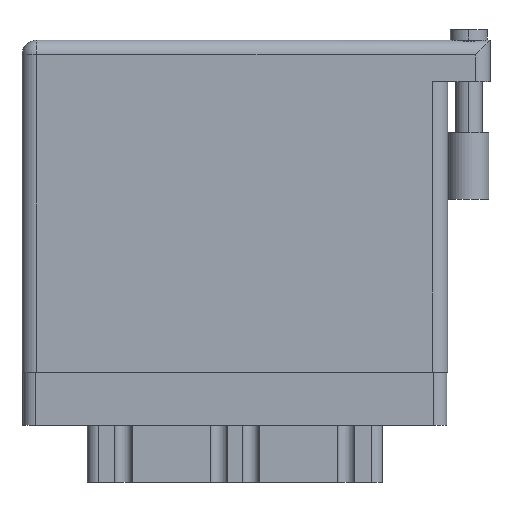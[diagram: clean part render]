
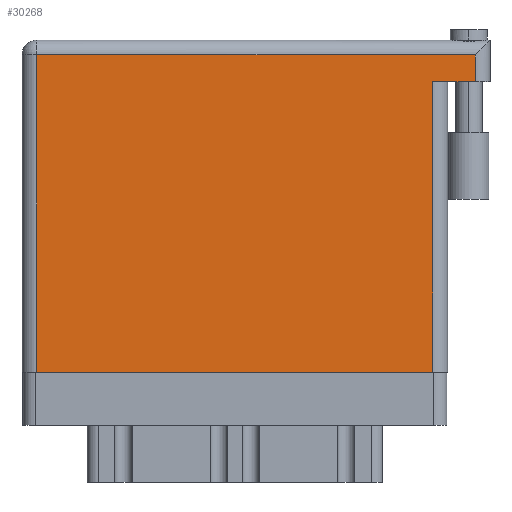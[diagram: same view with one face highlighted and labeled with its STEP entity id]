
A CAD part, front view. The second image highlights one B-rep face of the part: STEP entity #30268.
In plain terms, the highlighted face is planar.
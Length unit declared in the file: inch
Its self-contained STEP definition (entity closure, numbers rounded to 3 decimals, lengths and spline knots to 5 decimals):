
#124 = ORIENTED_EDGE ( 'NONE', *, *, #16181, .T. ) ;
#976 = DIRECTION ( 'NONE',  ( 0., 1., 0. ) ) ;
#1570 = VECTOR ( 'NONE', #4460, 39.37008 ) ;
#2046 = VECTOR ( 'NONE', #31741, 39.37008 ) ;
#2298 = LINE ( 'NONE', #10660, #4826 ) ;
#2504 = ORIENTED_EDGE ( 'NONE', *, *, #26879, .T. ) ;
#2647 = VERTEX_POINT ( 'NONE', #14250 ) ;
#3140 = ORIENTED_EDGE ( 'NONE', *, *, #25198, .T. ) ;
#3285 = VERTEX_POINT ( 'NONE', #3614 ) ;
#3614 = CARTESIAN_POINT ( 'NONE',  ( 2.138, 1.496, 0. ) ) ;
#4226 = EDGE_CURVE ( 'NONE', #24321, #3285, #29999, .T. ) ;
#4243 = CARTESIAN_POINT ( 'NONE',  ( 0., 1.566, 0. ) ) ;
#4258 = VERTEX_POINT ( 'NONE', #6030 ) ;
#4420 = DIRECTION ( 'NONE',  ( -1., 0., 0. ) ) ;
#4460 = DIRECTION ( 'NONE',  ( 1., 0., 0. ) ) ;
#4727 = CARTESIAN_POINT ( 'NONE',  ( 1.938, 1.369, 0. ) ) ;
#4826 = VECTOR ( 'NONE', #28879, 39.37008 ) ;
#6030 = CARTESIAN_POINT ( 'NONE',  ( 0.07, 0., 0. ) ) ;
#8004 = VECTOR ( 'NONE', #25530, 39.37008 ) ;
#8796 = EDGE_CURVE ( 'NONE', #24321, #25114, #18765, .T. ) ;
#9815 = DIRECTION ( 'NONE',  ( 0., 0., -1. ) ) ;
#9940 = EDGE_CURVE ( 'NONE', #13875, #4258, #13584, .T. ) ;
#10660 = CARTESIAN_POINT ( 'NONE',  ( 1.938, 1.369, 0. ) ) ;
#11923 = ORIENTED_EDGE ( 'NONE', *, *, #8796, .F. ) ;
#12043 = CARTESIAN_POINT ( 'NONE',  ( 0., 1.496, 0. ) ) ;
#13584 = LINE ( 'NONE', #17265, #20242 ) ;
#13875 = VERTEX_POINT ( 'NONE', #24393 ) ;
#14250 = CARTESIAN_POINT ( 'NONE',  ( 1.938, 0., 0. ) ) ;
#15868 = VECTOR ( 'NONE', #976, 39.37008 ) ;
#16181 = EDGE_CURVE ( 'NONE', #3285, #13875, #33427, .T. ) ;
#16619 = ORIENTED_EDGE ( 'NONE', *, *, #9940, .T. ) ;
#17026 = CARTESIAN_POINT ( 'NONE',  ( 2.138, 1.369, 0. ) ) ;
#17213 = CARTESIAN_POINT ( 'NONE',  ( 0., 0., 0. ) ) ;
#17265 = CARTESIAN_POINT ( 'NONE',  ( 0.07, 0., 0. ) ) ;
#17737 = LINE ( 'NONE', #17213, #1570 ) ;
#18345 = EDGE_LOOP ( 'NONE', ( #2504, #3140, #11923, #30069, #124, #16619 ) ) ;
#18765 = LINE ( 'NONE', #31550, #2046 ) ;
#19854 = AXIS2_PLACEMENT_3D ( 'NONE', #4243, #9815, #4420 ) ;
#20242 = VECTOR ( 'NONE', #27942, 39.37008 ) ;
#20295 = FACE_OUTER_BOUND ( 'NONE', #18345, .T. ) ;
#24321 = VERTEX_POINT ( 'NONE', #17026 ) ;
#24393 = CARTESIAN_POINT ( 'NONE',  ( 0.07, 1.496, 0. ) ) ;
#25114 = VERTEX_POINT ( 'NONE', #4727 ) ;
#25198 = EDGE_CURVE ( 'NONE', #2647, #25114, #2298, .T. ) ;
#25530 = DIRECTION ( 'NONE',  ( -1., 0., 0. ) ) ;
#26879 = EDGE_CURVE ( 'NONE', #4258, #2647, #17737, .T. ) ;
#27942 = DIRECTION ( 'NONE',  ( 0., -1., 0. ) ) ;
#28879 = DIRECTION ( 'NONE',  ( 0., 1., 0. ) ) ;
#29999 = LINE ( 'NONE', #30167, #15868 ) ;
#30069 = ORIENTED_EDGE ( 'NONE', *, *, #4226, .T. ) ;
#30167 = CARTESIAN_POINT ( 'NONE',  ( 2.138, 1.566, 0. ) ) ;
#30268 = ADVANCED_FACE ( 'NONE', ( #20295 ), #31343, .F. ) ;
#31343 = PLANE ( 'NONE',  #19854 ) ;
#31550 = CARTESIAN_POINT ( 'NONE',  ( 2.208, 1.369, 0. ) ) ;
#31741 = DIRECTION ( 'NONE',  ( -1., 0., 0. ) ) ;
#33427 = LINE ( 'NONE', #12043, #8004 ) ;
